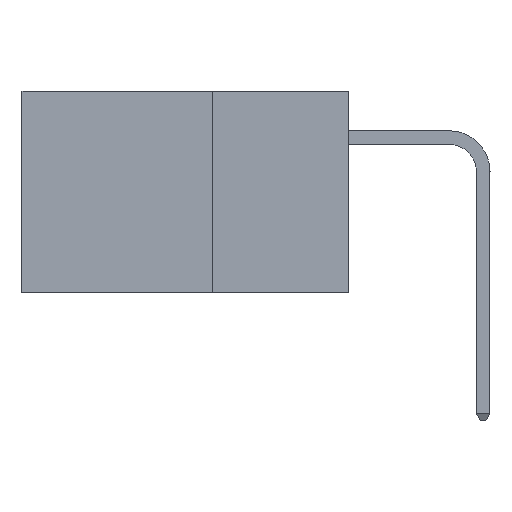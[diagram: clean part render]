
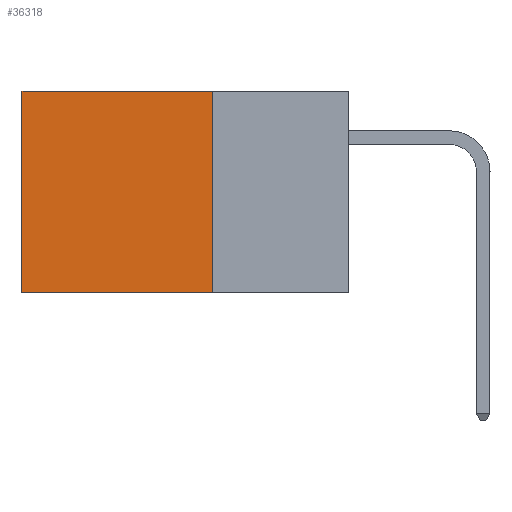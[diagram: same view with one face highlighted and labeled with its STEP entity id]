
A CAD part, left-side view. The second image highlights one B-rep face of the part: STEP entity #36318.
In plain terms, the highlighted planar face has unit normal (-1, 0, 0).
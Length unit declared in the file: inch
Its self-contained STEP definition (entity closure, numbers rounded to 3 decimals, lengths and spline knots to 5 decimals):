
#1793 = DIRECTION ( 'NONE',  ( 0., 0., -1. ) ) ;
#2383 = VECTOR ( 'NONE', #1793, 39.37008 ) ;
#3387 = VECTOR ( 'NONE', #16412, 39.37008 ) ;
#3404 = CARTESIAN_POINT ( 'NONE',  ( 0.2875, 0.6, 0. ) ) ;
#3644 = CARTESIAN_POINT ( 'NONE',  ( 0.2875, 0.25, -0.37 ) ) ;
#4828 = DIRECTION ( 'NONE',  ( 1., 0., 0. ) ) ;
#5196 = CARTESIAN_POINT ( 'NONE',  ( 0.2875, 0.25, 0. ) ) ;
#6347 = EDGE_LOOP ( 'NONE', ( #36826, #19679, #29200, #16223 ) ) ;
#9305 = DIRECTION ( 'NONE',  ( 0., 0., -1. ) ) ;
#10296 = VERTEX_POINT ( 'NONE', #18524 ) ;
#10881 = CARTESIAN_POINT ( 'NONE',  ( 0.2875, 0.6, -0.37 ) ) ;
#11111 = VERTEX_POINT ( 'NONE', #10881 ) ;
#11407 = VECTOR ( 'NONE', #21449, 39.37008 ) ;
#13508 = CARTESIAN_POINT ( 'NONE',  ( 0.2875, 0.25, -0.37 ) ) ;
#13564 = VERTEX_POINT ( 'NONE', #5196 ) ;
#14740 = EDGE_CURVE ( 'NONE', #26782, #11111, #26594, .T. ) ;
#15337 = AXIS2_PLACEMENT_3D ( 'NONE', #22247, #4828, #25145 ) ;
#16223 = ORIENTED_EDGE ( 'NONE', *, *, #17448, .T. ) ;
#16412 = DIRECTION ( 'NONE',  ( 0., 1., 0. ) ) ;
#16728 = LINE ( 'NONE', #3404, #22649 ) ;
#17448 = EDGE_CURVE ( 'NONE', #13564, #10296, #20943, .T. ) ;
#18524 = CARTESIAN_POINT ( 'NONE',  ( 0.2875, 0.6, 0. ) ) ;
#19252 = CARTESIAN_POINT ( 'NONE',  ( 0.2875, 0.25, 0. ) ) ;
#19679 = ORIENTED_EDGE ( 'NONE', *, *, #14740, .F. ) ;
#20607 = FACE_OUTER_BOUND ( 'NONE', #6347, .T. ) ;
#20943 = LINE ( 'NONE', #24362, #11407 ) ;
#21449 = DIRECTION ( 'NONE',  ( 0., 1., 0. ) ) ;
#22247 = CARTESIAN_POINT ( 'NONE',  ( 0.2875, 0.25, 0. ) ) ;
#22649 = VECTOR ( 'NONE', #9305, 39.37008 ) ;
#24362 = CARTESIAN_POINT ( 'NONE',  ( 0.2875, 0.25, 0. ) ) ;
#25145 = DIRECTION ( 'NONE',  ( 0., 0., -1. ) ) ;
#25592 = LINE ( 'NONE', #19252, #2383 ) ;
#25776 = EDGE_CURVE ( 'NONE', #13564, #26782, #25592, .T. ) ;
#26594 = LINE ( 'NONE', #13508, #3387 ) ;
#26782 = VERTEX_POINT ( 'NONE', #3644 ) ;
#29200 = ORIENTED_EDGE ( 'NONE', *, *, #25776, .F. ) ;
#32053 = EDGE_CURVE ( 'NONE', #10296, #11111, #16728, .T. ) ;
#36318 = ADVANCED_FACE ( 'NONE', ( #20607 ), #36666, .F. ) ;
#36666 = PLANE ( 'NONE',  #15337 ) ;
#36826 = ORIENTED_EDGE ( 'NONE', *, *, #32053, .T. ) ;
